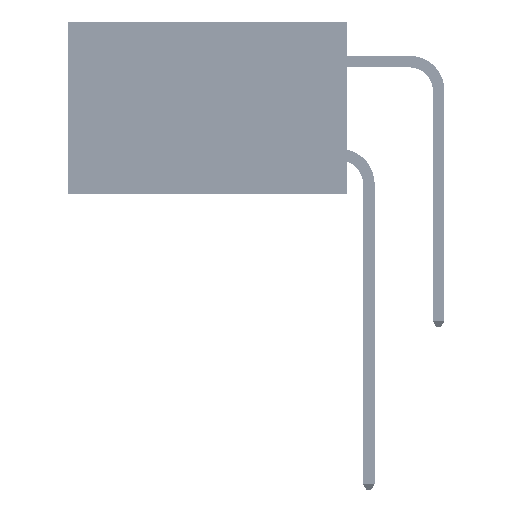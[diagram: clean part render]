
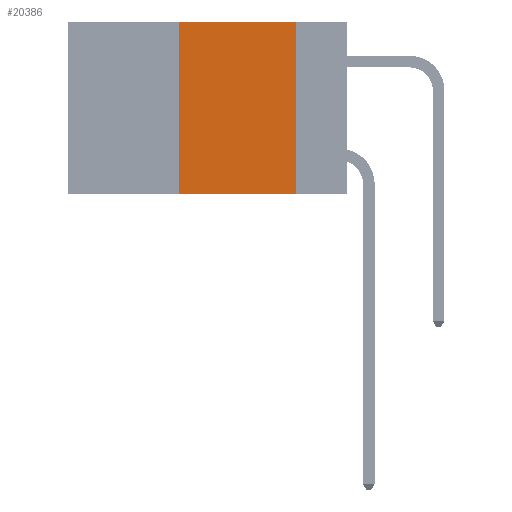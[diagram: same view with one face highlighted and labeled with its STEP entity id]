
A CAD part, left-side view. The second image highlights one B-rep face of the part: STEP entity #20386.
In plain terms, the highlighted planar face has unit normal (-1, 0, 0).
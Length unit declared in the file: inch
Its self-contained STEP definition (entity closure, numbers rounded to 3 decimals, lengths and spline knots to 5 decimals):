
#1953 = DIRECTION ( 'NONE',  ( 0., 0., -1. ) ) ;
#7273 = CARTESIAN_POINT ( 'NONE',  ( 0., 0.11, 0. ) ) ;
#7338 = VECTOR ( 'NONE', #28502, 39.37008 ) ;
#7526 = CARTESIAN_POINT ( 'NONE',  ( 0., 0.11, -0.37 ) ) ;
#10236 = LINE ( 'NONE', #29273, #20313 ) ;
#10641 = AXIS2_PLACEMENT_3D ( 'NONE', #35577, #24549, #1953 ) ;
#11211 = EDGE_CURVE ( 'NONE', #28313, #26903, #36947, .T. ) ;
#15052 = EDGE_CURVE ( 'NONE', #28313, #35625, #27372, .T. ) ;
#15184 = EDGE_CURVE ( 'NONE', #46148, #35625, #10236, .T. ) ;
#17237 = ORIENTED_EDGE ( 'NONE', *, *, #32248, .F. ) ;
#17631 = CARTESIAN_POINT ( 'NONE',  ( 0., 0.36, 0. ) ) ;
#18866 = FACE_OUTER_BOUND ( 'NONE', #39102, .T. ) ;
#20313 = VECTOR ( 'NONE', #47569, 39.37008 ) ;
#20386 = ADVANCED_FACE ( 'NONE', ( #18866 ), #20815, .F. ) ;
#20815 = PLANE ( 'NONE',  #10641 ) ;
#22836 = CARTESIAN_POINT ( 'NONE',  ( 0., 0.36, -0.37 ) ) ;
#24549 = DIRECTION ( 'NONE',  ( 1., 0., 0. ) ) ;
#25155 = DIRECTION ( 'NONE',  ( 0., 0., 1. ) ) ;
#26234 = CARTESIAN_POINT ( 'NONE',  ( 0., 0.6, 0. ) ) ;
#26903 = VERTEX_POINT ( 'NONE', #28556 ) ;
#27087 = LINE ( 'NONE', #26234, #45485 ) ;
#27372 = LINE ( 'NONE', #46800, #7338 ) ;
#28313 = VERTEX_POINT ( 'NONE', #22836 ) ;
#28502 = DIRECTION ( 'NONE',  ( 0., -1., 0. ) ) ;
#28556 = CARTESIAN_POINT ( 'NONE',  ( 0., 0.36, 0. ) ) ;
#29273 = CARTESIAN_POINT ( 'NONE',  ( 0., 0.11, 0. ) ) ;
#29976 = DIRECTION ( 'NONE',  ( 0., -1., 0. ) ) ;
#32248 = EDGE_CURVE ( 'NONE', #26903, #46148, #27087, .T. ) ;
#34135 = ORIENTED_EDGE ( 'NONE', *, *, #11211, .F. ) ;
#35577 = CARTESIAN_POINT ( 'NONE',  ( 0., 0.6, 0. ) ) ;
#35625 = VERTEX_POINT ( 'NONE', #7526 ) ;
#36947 = LINE ( 'NONE', #17631, #45548 ) ;
#37589 = ORIENTED_EDGE ( 'NONE', *, *, #15052, .T. ) ;
#39102 = EDGE_LOOP ( 'NONE', ( #47236, #17237, #34135, #37589 ) ) ;
#45485 = VECTOR ( 'NONE', #29976, 39.37008 ) ;
#45548 = VECTOR ( 'NONE', #25155, 39.37008 ) ;
#46148 = VERTEX_POINT ( 'NONE', #7273 ) ;
#46800 = CARTESIAN_POINT ( 'NONE',  ( 0., 0.6, -0.37 ) ) ;
#47236 = ORIENTED_EDGE ( 'NONE', *, *, #15184, .F. ) ;
#47569 = DIRECTION ( 'NONE',  ( 0., 0., -1. ) ) ;
